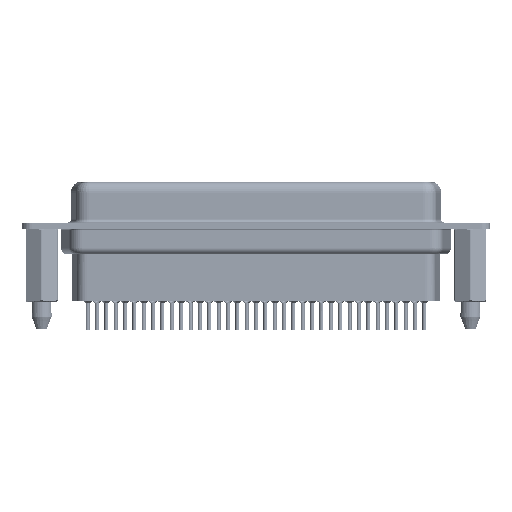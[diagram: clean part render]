
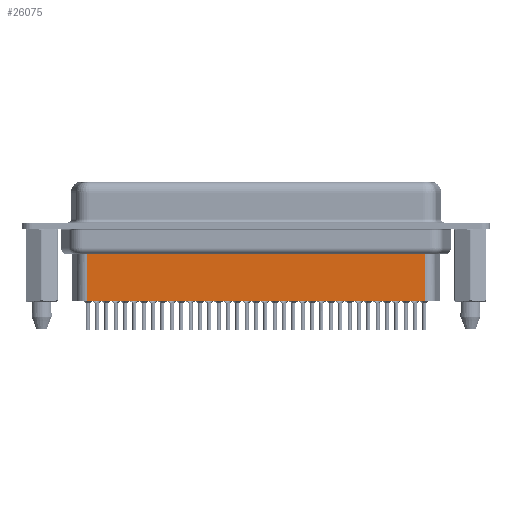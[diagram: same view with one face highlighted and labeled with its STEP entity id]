
A CAD part, front view. The second image highlights one B-rep face of the part: STEP entity #26075.
In plain terms, the highlighted planar face has unit normal (0, -1, 0).
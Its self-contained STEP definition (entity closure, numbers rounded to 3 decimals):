
#563 = LINE ( 'NONE', #11785, #23577 ) ;
#1209 = VECTOR ( 'NONE', #14193, 1000. ) ;
#1878 = CARTESIAN_POINT ( 'NONE',  ( 6.706, -3.5, -3.1 ) ) ;
#2190 = ORIENTED_EDGE ( 'NONE', *, *, #11730, .T. ) ;
#3583 = DIRECTION ( 'NONE',  ( -1., 0., 0. ) ) ;
#4571 = CARTESIAN_POINT ( 'NONE',  ( 56.794, -3.5, -4.097 ) ) ;
#4636 = DIRECTION ( 'NONE',  ( 1., 0., 0. ) ) ;
#5459 = VECTOR ( 'NONE', #3583, 1000. ) ;
#6090 = CARTESIAN_POINT ( 'NONE',  ( 6.706, -3.5, -4.097 ) ) ;
#6700 = VERTEX_POINT ( 'NONE', #4571 ) ;
#6888 = CARTESIAN_POINT ( 'NONE',  ( 6.459, -3.5, -4.097 ) ) ;
#7062 = AXIS2_PLACEMENT_3D ( 'NONE', #1878, #21585, #4636 ) ;
#8400 = EDGE_CURVE ( 'NONE', #17998, #13692, #24136, .T. ) ;
#9466 = LINE ( 'NONE', #6888, #5459 ) ;
#9798 = CARTESIAN_POINT ( 'NONE',  ( 56.794, -3.5, -11.15 ) ) ;
#9972 = FACE_OUTER_BOUND ( 'NONE', #20030, .T. ) ;
#10929 = ORIENTED_EDGE ( 'NONE', *, *, #30800, .T. ) ;
#11713 = EDGE_CURVE ( 'NONE', #6700, #17998, #563, .T. ) ;
#11730 = EDGE_CURVE ( 'NONE', #18215, #13692, #20629, .T. ) ;
#11785 = CARTESIAN_POINT ( 'NONE',  ( 56.794, -3.5, -3.1 ) ) ;
#13057 = DIRECTION ( 'NONE',  ( -1., 0., 0. ) ) ;
#13692 = VERTEX_POINT ( 'NONE', #30273 ) ;
#14193 = DIRECTION ( 'NONE',  ( 0., 0., -1. ) ) ;
#15092 = ORIENTED_EDGE ( 'NONE', *, *, #8400, .F. ) ;
#16062 = ORIENTED_EDGE ( 'NONE', *, *, #11713, .F. ) ;
#17998 = VERTEX_POINT ( 'NONE', #9798 ) ;
#18215 = VERTEX_POINT ( 'NONE', #6090 ) ;
#20030 = EDGE_LOOP ( 'NONE', ( #16062, #10929, #2190, #15092 ) ) ;
#20629 = LINE ( 'NONE', #28218, #1209 ) ;
#21585 = DIRECTION ( 'NONE',  ( 0., -1., 0. ) ) ;
#23577 = VECTOR ( 'NONE', #28383, 1000. ) ;
#24136 = LINE ( 'NONE', #29131, #28725 ) ;
#26075 = ADVANCED_FACE ( 'NONE', ( #9972 ), #35939, .T. ) ;
#28218 = CARTESIAN_POINT ( 'NONE',  ( 6.706, -3.5, -3.1 ) ) ;
#28383 = DIRECTION ( 'NONE',  ( 0., 0., -1. ) ) ;
#28725 = VECTOR ( 'NONE', #13057, 1000. ) ;
#29131 = CARTESIAN_POINT ( 'NONE',  ( 6.706, -3.5, -11.15 ) ) ;
#30273 = CARTESIAN_POINT ( 'NONE',  ( 6.706, -3.5, -11.15 ) ) ;
#30800 = EDGE_CURVE ( 'NONE', #6700, #18215, #9466, .T. ) ;
#35939 = PLANE ( 'NONE',  #7062 ) ;
